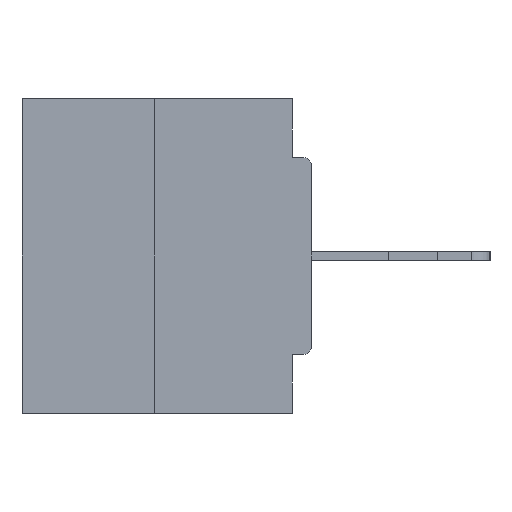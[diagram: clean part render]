
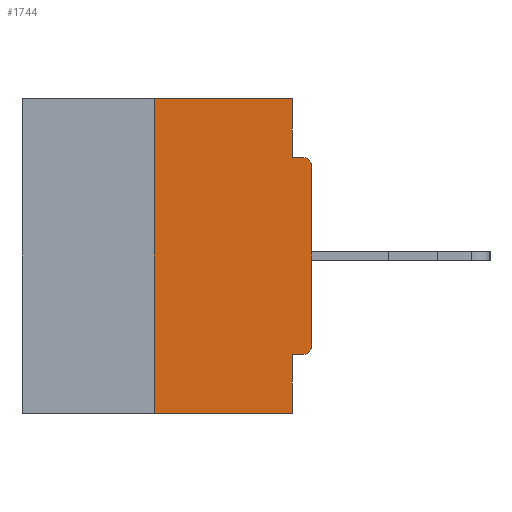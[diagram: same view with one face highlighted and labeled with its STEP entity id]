
A CAD part, left-side view. The second image highlights one B-rep face of the part: STEP entity #1744.
In plain terms, the highlighted planar face has unit normal (-1, 0, 0).
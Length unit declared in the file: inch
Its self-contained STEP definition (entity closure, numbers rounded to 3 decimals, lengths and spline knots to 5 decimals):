
#291 = FACE_OUTER_BOUND ( 'NONE', #19529, .T. ) ;
#379 = LINE ( 'NONE', #28644, #16320 ) ;
#502 = CARTESIAN_POINT ( 'NONE',  ( 0., 0.015, -0.3915 ) ) ;
#545 = LINE ( 'NONE', #26608, #10742 ) ;
#661 = LINE ( 'NONE', #24316, #29168 ) ;
#732 = ORIENTED_EDGE ( 'NONE', *, *, #9101, .F. ) ;
#1744 = ADVANCED_FACE ( 'NONE', ( #291 ), #15841, .F. ) ;
#1752 = VECTOR ( 'NONE', #30023, 39.37008 ) ;
#1996 = VECTOR ( 'NONE', #14782, 39.37008 ) ;
#2251 = EDGE_CURVE ( 'NONE', #27326, #15550, #3521, .T. ) ;
#3353 = VERTEX_POINT ( 'NONE', #13548 ) ;
#3521 = LINE ( 'NONE', #29936, #23726 ) ;
#3795 = LINE ( 'NONE', #14144, #1752 ) ;
#4403 = CARTESIAN_POINT ( 'NONE',  ( 0., 0.015, -0.4065 ) ) ;
#5302 = DIRECTION ( 'NONE',  ( 0., 0., -1. ) ) ;
#5549 = ORIENTED_EDGE ( 'NONE', *, *, #20256, .T. ) ;
#5711 = LINE ( 'NONE', #16593, #23311 ) ;
#6895 = VERTEX_POINT ( 'NONE', #29112 ) ;
#8380 = ORIENTED_EDGE ( 'NONE', *, *, #22224, .F. ) ;
#9101 = EDGE_CURVE ( 'NONE', #21085, #23587, #379, .T. ) ;
#9415 = CARTESIAN_POINT ( 'NONE',  ( 0., 0., -0.4065 ) ) ;
#9446 = EDGE_CURVE ( 'NONE', #17214, #30891, #22723, .T. ) ;
#9855 = ORIENTED_EDGE ( 'NONE', *, *, #9446, .F. ) ;
#10286 = VERTEX_POINT ( 'NONE', #25185 ) ;
#10688 = AXIS2_PLACEMENT_3D ( 'NONE', #29355, #29195, #26614 ) ;
#10717 = DIRECTION ( 'NONE',  ( 0., 0., 1. ) ) ;
#10742 = VECTOR ( 'NONE', #15728, 39.37008 ) ;
#12016 = EDGE_CURVE ( 'NONE', #23587, #32971, #3795, .T. ) ;
#12457 = ORIENTED_EDGE ( 'NONE', *, *, #33706, .F. ) ;
#13197 = CIRCLE ( 'NONE', #24776, 0.015 ) ;
#13548 = CARTESIAN_POINT ( 'NONE',  ( 0., 0., -0.3915 ) ) ;
#13623 = DIRECTION ( 'NONE',  ( -1., 0., 0. ) ) ;
#14144 = CARTESIAN_POINT ( 'NONE',  ( 0., 0.031, 0. ) ) ;
#14234 = DIRECTION ( 'NONE',  ( 0., -1., 0. ) ) ;
#14449 = CARTESIAN_POINT ( 'NONE',  ( 0., 0.031, -0.5 ) ) ;
#14782 = DIRECTION ( 'NONE',  ( 0., -1., 0. ) ) ;
#15248 = AXIS2_PLACEMENT_3D ( 'NONE', #18425, #28941, #5302 ) ;
#15550 = VERTEX_POINT ( 'NONE', #14449 ) ;
#15728 = DIRECTION ( 'NONE',  ( 0., 0., 1. ) ) ;
#15841 = PLANE ( 'NONE',  #15248 ) ;
#16320 = VECTOR ( 'NONE', #31052, 39.37008 ) ;
#16593 = CARTESIAN_POINT ( 'NONE',  ( 0., 0., 0. ) ) ;
#16594 = EDGE_CURVE ( 'NONE', #27326, #21085, #545, .T. ) ;
#17214 = VERTEX_POINT ( 'NONE', #4403 ) ;
#17531 = ORIENTED_EDGE ( 'NONE', *, *, #16594, .F. ) ;
#18425 = CARTESIAN_POINT ( 'NONE',  ( 0., 0.46, 0. ) ) ;
#19529 = EDGE_LOOP ( 'NONE', ( #732, #17531, #27654, #12457, #9855, #32108, #22520, #5549, #8380, #29498 ) ) ;
#20211 = VECTOR ( 'NONE', #22381, 39.37008 ) ;
#20256 = EDGE_CURVE ( 'NONE', #6895, #10286, #21186, .T. ) ;
#21085 = VERTEX_POINT ( 'NONE', #30827 ) ;
#21186 = CIRCLE ( 'NONE', #10688, 0.015 ) ;
#22224 = EDGE_CURVE ( 'NONE', #32971, #10286, #27559, .T. ) ;
#22381 = DIRECTION ( 'NONE',  ( 0., 1., 0. ) ) ;
#22520 = ORIENTED_EDGE ( 'NONE', *, *, #22928, .T. ) ;
#22723 = LINE ( 'NONE', #9415, #20211 ) ;
#22928 = EDGE_CURVE ( 'NONE', #3353, #6895, #5711, .T. ) ;
#23311 = VECTOR ( 'NONE', #10717, 39.37008 ) ;
#23390 = CARTESIAN_POINT ( 'NONE',  ( 0., 0.031, 0. ) ) ;
#23587 = VERTEX_POINT ( 'NONE', #23390 ) ;
#23726 = VECTOR ( 'NONE', #14234, 39.37008 ) ;
#24316 = CARTESIAN_POINT ( 'NONE',  ( 0., 0.031, -0.5 ) ) ;
#24348 = CARTESIAN_POINT ( 'NONE',  ( 0., 0.031, -0.4065 ) ) ;
#24776 = AXIS2_PLACEMENT_3D ( 'NONE', #502, #13623, #29302 ) ;
#25185 = CARTESIAN_POINT ( 'NONE',  ( 0., 0.015, -0.0935 ) ) ;
#25846 = CARTESIAN_POINT ( 'NONE',  ( 0., 0.25, -0.5 ) ) ;
#26608 = CARTESIAN_POINT ( 'NONE',  ( 0., 0.25, 0. ) ) ;
#26614 = DIRECTION ( 'NONE',  ( 0., 0., -1. ) ) ;
#27326 = VERTEX_POINT ( 'NONE', #25846 ) ;
#27559 = LINE ( 'NONE', #32907, #1996 ) ;
#27654 = ORIENTED_EDGE ( 'NONE', *, *, #2251, .T. ) ;
#28644 = CARTESIAN_POINT ( 'NONE',  ( 0., 0.46, 0. ) ) ;
#28941 = DIRECTION ( 'NONE',  ( 1., 0., 0. ) ) ;
#29112 = CARTESIAN_POINT ( 'NONE',  ( 0., 0., -0.1085 ) ) ;
#29168 = VECTOR ( 'NONE', #32600, 39.37008 ) ;
#29195 = DIRECTION ( 'NONE',  ( -1., 0., 0. ) ) ;
#29302 = DIRECTION ( 'NONE',  ( 0., 0., -1. ) ) ;
#29355 = CARTESIAN_POINT ( 'NONE',  ( 0., 0.015, -0.1085 ) ) ;
#29498 = ORIENTED_EDGE ( 'NONE', *, *, #12016, .F. ) ;
#29936 = CARTESIAN_POINT ( 'NONE',  ( 0., 0.46, -0.5 ) ) ;
#30023 = DIRECTION ( 'NONE',  ( 0., 0., -1. ) ) ;
#30827 = CARTESIAN_POINT ( 'NONE',  ( 0., 0.25, 0. ) ) ;
#30891 = VERTEX_POINT ( 'NONE', #24348 ) ;
#31052 = DIRECTION ( 'NONE',  ( 0., -1., 0. ) ) ;
#32108 = ORIENTED_EDGE ( 'NONE', *, *, #33748, .T. ) ;
#32600 = DIRECTION ( 'NONE',  ( 0., 0., -1. ) ) ;
#32838 = CARTESIAN_POINT ( 'NONE',  ( 0., 0.031, -0.0935 ) ) ;
#32907 = CARTESIAN_POINT ( 'NONE',  ( 0., 0., -0.0935 ) ) ;
#32971 = VERTEX_POINT ( 'NONE', #32838 ) ;
#33706 = EDGE_CURVE ( 'NONE', #30891, #15550, #661, .T. ) ;
#33748 = EDGE_CURVE ( 'NONE', #17214, #3353, #13197, .T. ) ;
